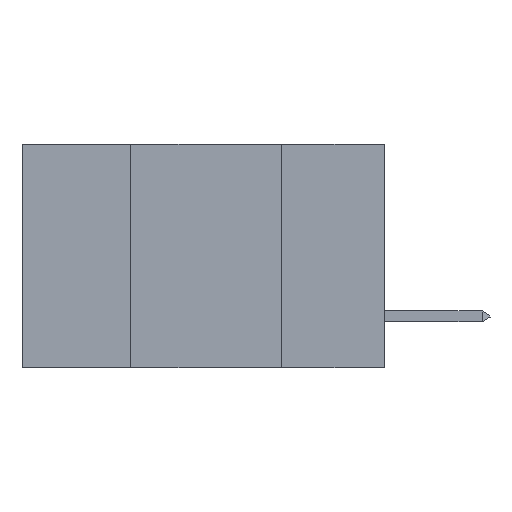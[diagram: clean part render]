
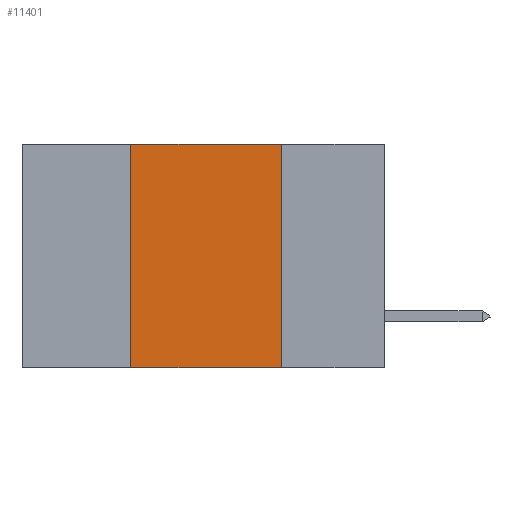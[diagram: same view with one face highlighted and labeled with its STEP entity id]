
A CAD part, left-side view. The second image highlights one B-rep face of the part: STEP entity #11401.
In plain terms, the highlighted planar face has unit normal (-1, 0, 0).
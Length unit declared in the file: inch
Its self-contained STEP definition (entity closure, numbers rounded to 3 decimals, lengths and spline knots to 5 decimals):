
#376 = LINE ( 'NONE', #4324, #2764 ) ;
#590 = VECTOR ( 'NONE', #2905, 39.37008 ) ;
#624 = ORIENTED_EDGE ( 'NONE', *, *, #5298, .F. ) ;
#2388 = DIRECTION ( 'NONE',  ( 0., 0., -1. ) ) ;
#2764 = VECTOR ( 'NONE', #16177, 39.37008 ) ;
#2905 = DIRECTION ( 'NONE',  ( 0., -1., 0. ) ) ;
#4324 = CARTESIAN_POINT ( 'NONE',  ( 0., 0.6, 0. ) ) ;
#4591 = LINE ( 'NONE', #19518, #14094 ) ;
#4680 = ORIENTED_EDGE ( 'NONE', *, *, #18974, .T. ) ;
#5298 = EDGE_CURVE ( 'NONE', #19110, #16134, #18110, .T. ) ;
#7657 = VERTEX_POINT ( 'NONE', #18636 ) ;
#7894 = ORIENTED_EDGE ( 'NONE', *, *, #8937, .F. ) ;
#8087 = CARTESIAN_POINT ( 'NONE',  ( 0., 0.6, -0.37 ) ) ;
#8673 = EDGE_LOOP ( 'NONE', ( #624, #7894, #12116, #4680 ) ) ;
#8937 = EDGE_CURVE ( 'NONE', #7657, #19110, #376, .T. ) ;
#9969 = CARTESIAN_POINT ( 'NONE',  ( 0., 0.17, 0. ) ) ;
#10468 = EDGE_CURVE ( 'NONE', #17044, #7657, #4591, .T. ) ;
#10719 = PLANE ( 'NONE',  #16116 ) ;
#11191 = LINE ( 'NONE', #8087, #590 ) ;
#11401 = ADVANCED_FACE ( 'NONE', ( #14841 ), #10719, .F. ) ;
#12015 = DIRECTION ( 'NONE',  ( 0., 0., -1. ) ) ;
#12116 = ORIENTED_EDGE ( 'NONE', *, *, #10468, .F. ) ;
#12233 = CARTESIAN_POINT ( 'NONE',  ( 0., 0.6, 0. ) ) ;
#12256 = CARTESIAN_POINT ( 'NONE',  ( 0., 0.17, -0.37 ) ) ;
#12882 = DIRECTION ( 'NONE',  ( 0., 0., 1. ) ) ;
#13641 = CARTESIAN_POINT ( 'NONE',  ( 0., 0.17, 0. ) ) ;
#14094 = VECTOR ( 'NONE', #12882, 39.37008 ) ;
#14679 = VECTOR ( 'NONE', #12015, 39.37008 ) ;
#14841 = FACE_OUTER_BOUND ( 'NONE', #8673, .T. ) ;
#16116 = AXIS2_PLACEMENT_3D ( 'NONE', #12233, #19155, #2388 ) ;
#16134 = VERTEX_POINT ( 'NONE', #12256 ) ;
#16177 = DIRECTION ( 'NONE',  ( 0., -1., 0. ) ) ;
#17044 = VERTEX_POINT ( 'NONE', #21289 ) ;
#18110 = LINE ( 'NONE', #13641, #14679 ) ;
#18636 = CARTESIAN_POINT ( 'NONE',  ( 0., 0.42, 0. ) ) ;
#18974 = EDGE_CURVE ( 'NONE', #17044, #16134, #11191, .T. ) ;
#19110 = VERTEX_POINT ( 'NONE', #9969 ) ;
#19155 = DIRECTION ( 'NONE',  ( 1., 0., 0. ) ) ;
#19518 = CARTESIAN_POINT ( 'NONE',  ( 0., 0.42, 0. ) ) ;
#21289 = CARTESIAN_POINT ( 'NONE',  ( 0., 0.42, -0.37 ) ) ;
